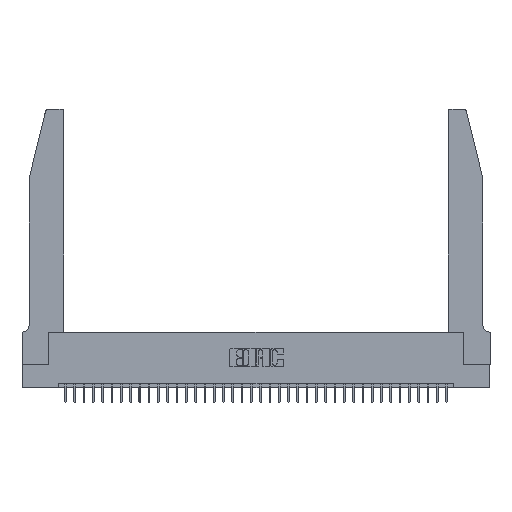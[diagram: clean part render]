
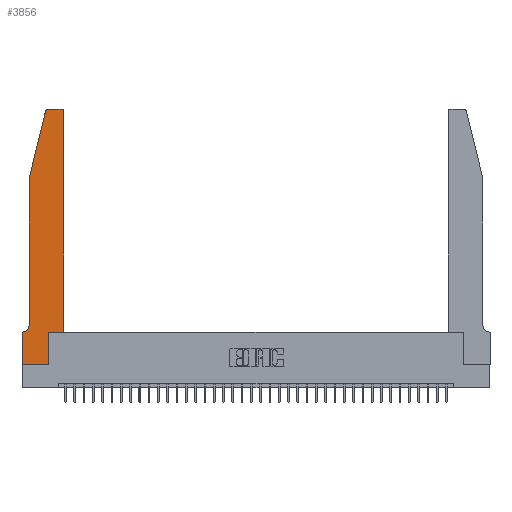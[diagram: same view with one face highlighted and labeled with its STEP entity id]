
A CAD part, top view. The second image highlights one B-rep face of the part: STEP entity #3856.
In plain terms, the highlighted planar face has unit normal (0, 0, 1).
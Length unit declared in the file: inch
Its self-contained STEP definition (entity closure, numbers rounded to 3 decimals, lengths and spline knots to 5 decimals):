
#505 = EDGE_CURVE ( 'NONE', #21991, #12345, #27936, .T. ) ;
#570 = DIRECTION ( 'NONE',  ( 1., 0., 0. ) ) ;
#639 = DIRECTION ( 'NONE',  ( 0., 0., 1. ) ) ;
#1433 = EDGE_LOOP ( 'NONE', ( #4450, #14062, #34469, #19279, #22554, #34308, #9678, #7873, #22074, #14521, #5875, #22570 ) ) ;
#1542 = CIRCLE ( 'NONE', #15149, 0.07 ) ;
#3262 = CARTESIAN_POINT ( 'NONE',  ( 0.4505, 0.35, 0.37 ) ) ;
#3737 = CARTESIAN_POINT ( 'NONE',  ( 0.0755, 2., 0.37 ) ) ;
#3856 = ADVANCED_FACE ( 'NONE', ( #17117 ), #18379, .T. ) ;
#3890 = LINE ( 'NONE', #28553, #10738 ) ;
#4450 = ORIENTED_EDGE ( 'NONE', *, *, #21129, .T. ) ;
#5204 = DIRECTION ( 'NONE',  ( 0., -1., 0. ) ) ;
#5875 = ORIENTED_EDGE ( 'NONE', *, *, #11785, .T. ) ;
#6041 = EDGE_CURVE ( 'NONE', #15757, #35165, #7777, .T. ) ;
#6639 = DIRECTION ( 'NONE',  ( -1., 0., 0. ) ) ;
#7410 = AXIS2_PLACEMENT_3D ( 'NONE', #18176, #639, #21095 ) ;
#7777 = CIRCLE ( 'NONE', #7410, 0.03 ) ;
#7873 = ORIENTED_EDGE ( 'NONE', *, *, #25762, .T. ) ;
#8009 = CARTESIAN_POINT ( 'NONE',  ( 0.4205, 2.75, 0.37 ) ) ;
#8170 = DIRECTION ( 'NONE',  ( -1., 0., 0. ) ) ;
#8472 = CARTESIAN_POINT ( 'NONE',  ( 0.2865, 0., 0.37 ) ) ;
#9281 = DIRECTION ( 'NONE',  ( 0., -1., 0. ) ) ;
#9664 = DIRECTION ( 'NONE',  ( 0., 0., 1. ) ) ;
#9678 = ORIENTED_EDGE ( 'NONE', *, *, #11627, .T. ) ;
#10038 = DIRECTION ( 'NONE',  ( 1., 0., 0. ) ) ;
#10089 = CARTESIAN_POINT ( 'NONE',  ( 0., 0.35, 0.37 ) ) ;
#10379 = AXIS2_PLACEMENT_3D ( 'NONE', #15120, #35462, #18072 ) ;
#10738 = VECTOR ( 'NONE', #5204, 39.37008 ) ;
#11627 = EDGE_CURVE ( 'NONE', #23128, #23870, #17655, .T. ) ;
#11628 = CARTESIAN_POINT ( 'NONE',  ( 0.0055, 0.42, 0.37 ) ) ;
#11785 = EDGE_CURVE ( 'NONE', #34309, #15757, #27663, .T. ) ;
#12345 = VERTEX_POINT ( 'NONE', #3737 ) ;
#12797 = EDGE_CURVE ( 'NONE', #13662, #17908, #1542, .T. ) ;
#13607 = CARTESIAN_POINT ( 'NONE',  ( 0.25487, 2.72718, 0.37 ) ) ;
#13662 = VERTEX_POINT ( 'NONE', #15391 ) ;
#14062 = ORIENTED_EDGE ( 'NONE', *, *, #24488, .T. ) ;
#14521 = ORIENTED_EDGE ( 'NONE', *, *, #25888, .T. ) ;
#14555 = DIRECTION ( 'NONE',  ( -1., 0., 0. ) ) ;
#14661 = LINE ( 'NONE', #21060, #36977 ) ;
#14769 = CARTESIAN_POINT ( 'NONE',  ( 0.4505, 2.72, 0.37 ) ) ;
#15120 = CARTESIAN_POINT ( 'NONE',  ( 0.284, 2.72, 0.37 ) ) ;
#15149 = AXIS2_PLACEMENT_3D ( 'NONE', #11628, #32010, #14555 ) ;
#15391 = CARTESIAN_POINT ( 'NONE',  ( 0.0755, 0.42, 0.37 ) ) ;
#15740 = VECTOR ( 'NONE', #570, 39.37008 ) ;
#15757 = VERTEX_POINT ( 'NONE', #14769 ) ;
#16291 = VERTEX_POINT ( 'NONE', #8472 ) ;
#17117 = FACE_OUTER_BOUND ( 'NONE', #1433, .T. ) ;
#17655 = LINE ( 'NONE', #26771, #18589 ) ;
#17850 = CARTESIAN_POINT ( 'NONE',  ( 0., 0., 0.37 ) ) ;
#17883 = CARTESIAN_POINT ( 'NONE',  ( 0.2865, 0.35, 0.37 ) ) ;
#17908 = VERTEX_POINT ( 'NONE', #21600 ) ;
#18072 = DIRECTION ( 'NONE',  ( 1., 0., 0. ) ) ;
#18107 = LINE ( 'NONE', #22729, #25852 ) ;
#18176 = CARTESIAN_POINT ( 'NONE',  ( 0.4205, 2.72, 0.37 ) ) ;
#18379 = PLANE ( 'NONE',  #23539 ) ;
#18589 = VECTOR ( 'NONE', #9281, 39.37008 ) ;
#19279 = ORIENTED_EDGE ( 'NONE', *, *, #25606, .T. ) ;
#19280 = VECTOR ( 'NONE', #22996, 39.37008 ) ;
#19803 = VERTEX_POINT ( 'NONE', #22217 ) ;
#19918 = VECTOR ( 'NONE', #24347, 39.37008 ) ;
#21060 = CARTESIAN_POINT ( 'NONE',  ( 0.2865, 0.35, 0.37 ) ) ;
#21095 = DIRECTION ( 'NONE',  ( 1., 0., 0. ) ) ;
#21129 = EDGE_CURVE ( 'NONE', #35165, #19803, #30784, .T. ) ;
#21600 = CARTESIAN_POINT ( 'NONE',  ( 0.0055, 0.35, 0.37 ) ) ;
#21991 = VERTEX_POINT ( 'NONE', #13607 ) ;
#22074 = ORIENTED_EDGE ( 'NONE', *, *, #36667, .T. ) ;
#22217 = CARTESIAN_POINT ( 'NONE',  ( 0.284, 2.75, 0.37 ) ) ;
#22554 = ORIENTED_EDGE ( 'NONE', *, *, #12797, .T. ) ;
#22570 = ORIENTED_EDGE ( 'NONE', *, *, #6041, .T. ) ;
#22729 = CARTESIAN_POINT ( 'NONE',  ( 0.0755, 0.35, 0.37 ) ) ;
#22996 = DIRECTION ( 'NONE',  ( -0.239, -0.971, 0. ) ) ;
#23128 = VERTEX_POINT ( 'NONE', #10089 ) ;
#23539 = AXIS2_PLACEMENT_3D ( 'NONE', #27180, #9664, #30076 ) ;
#23870 = VERTEX_POINT ( 'NONE', #17850 ) ;
#24347 = DIRECTION ( 'NONE',  ( 0., 1., 0. ) ) ;
#24488 = EDGE_CURVE ( 'NONE', #19803, #21991, #32709, .T. ) ;
#24919 = EDGE_CURVE ( 'NONE', #17908, #23128, #18107, .T. ) ;
#25164 = VERTEX_POINT ( 'NONE', #17883 ) ;
#25606 = EDGE_CURVE ( 'NONE', #12345, #13662, #3890, .T. ) ;
#25762 = EDGE_CURVE ( 'NONE', #23870, #16291, #30332, .T. ) ;
#25852 = VECTOR ( 'NONE', #8170, 39.37008 ) ;
#25888 = EDGE_CURVE ( 'NONE', #25164, #34309, #33524, .T. ) ;
#26771 = CARTESIAN_POINT ( 'NONE',  ( 0., 0., 0.37 ) ) ;
#27180 = CARTESIAN_POINT ( 'NONE',  ( 0., 0.35, 0.37 ) ) ;
#27663 = LINE ( 'NONE', #35889, #19918 ) ;
#27936 = LINE ( 'NONE', #28846, #19280 ) ;
#28553 = CARTESIAN_POINT ( 'NONE',  ( 0.0755, 2., 0.37 ) ) ;
#28846 = CARTESIAN_POINT ( 'NONE',  ( 0.0755, 2., 0.37 ) ) ;
#28966 = VECTOR ( 'NONE', #6639, 39.37008 ) ;
#29853 = DIRECTION ( 'NONE',  ( 0., 1., 0. ) ) ;
#30076 = DIRECTION ( 'NONE',  ( 1., 0., 0. ) ) ;
#30332 = LINE ( 'NONE', #35513, #15740 ) ;
#30784 = LINE ( 'NONE', #35812, #28966 ) ;
#31689 = VECTOR ( 'NONE', #10038, 39.37008 ) ;
#32010 = DIRECTION ( 'NONE',  ( 0., 0., -1. ) ) ;
#32709 = CIRCLE ( 'NONE', #10379, 0.03 ) ;
#33379 = CARTESIAN_POINT ( 'NONE',  ( 0.4505, 0.35, 0.37 ) ) ;
#33524 = LINE ( 'NONE', #33379, #31689 ) ;
#34308 = ORIENTED_EDGE ( 'NONE', *, *, #24919, .T. ) ;
#34309 = VERTEX_POINT ( 'NONE', #3262 ) ;
#34469 = ORIENTED_EDGE ( 'NONE', *, *, #505, .T. ) ;
#35165 = VERTEX_POINT ( 'NONE', #8009 ) ;
#35462 = DIRECTION ( 'NONE',  ( 0., 0., 1. ) ) ;
#35513 = CARTESIAN_POINT ( 'NONE',  ( 0., 0., 0.37 ) ) ;
#35812 = CARTESIAN_POINT ( 'NONE',  ( 0.2605, 2.75, 0.37 ) ) ;
#35889 = CARTESIAN_POINT ( 'NONE',  ( 0.4505, 0.35, 0.37 ) ) ;
#36667 = EDGE_CURVE ( 'NONE', #16291, #25164, #14661, .T. ) ;
#36977 = VECTOR ( 'NONE', #29853, 39.37008 ) ;
